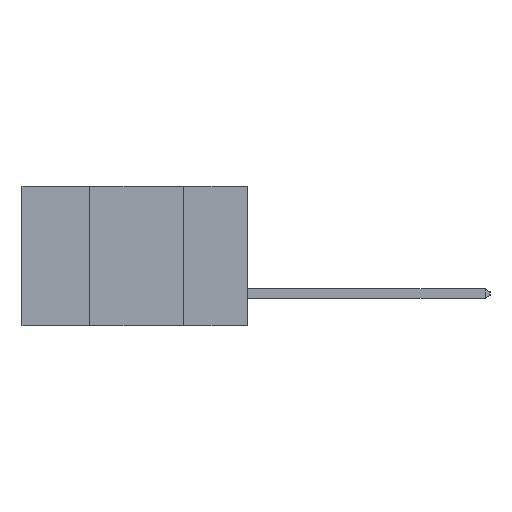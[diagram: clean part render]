
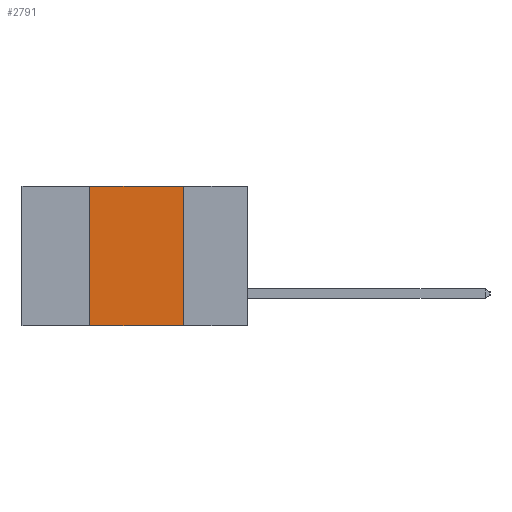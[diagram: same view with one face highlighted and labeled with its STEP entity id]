
A CAD part, left-side view. The second image highlights one B-rep face of the part: STEP entity #2791.
In plain terms, the highlighted planar face has unit normal (-1, 0, 0).
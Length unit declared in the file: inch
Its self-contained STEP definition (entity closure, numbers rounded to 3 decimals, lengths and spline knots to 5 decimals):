
#1742 = CARTESIAN_POINT ( 'NONE',  ( 0., 0.6, 0. ) ) ;
#1952 = ORIENTED_EDGE ( 'NONE', *, *, #18588, .F. ) ;
#2791 = ADVANCED_FACE ( 'NONE', ( #20712 ), #13685, .F. ) ;
#3406 = LINE ( 'NONE', #10914, #11964 ) ;
#4658 = EDGE_CURVE ( 'NONE', #15709, #16392, #15231, .T. ) ;
#6095 = EDGE_CURVE ( 'NONE', #9478, #14396, #9976, .T. ) ;
#6897 = CARTESIAN_POINT ( 'NONE',  ( 0., 0.42, -0.37 ) ) ;
#7161 = DIRECTION ( 'NONE',  ( 0., 0., -1. ) ) ;
#7363 = ORIENTED_EDGE ( 'NONE', *, *, #6095, .F. ) ;
#7579 = CARTESIAN_POINT ( 'NONE',  ( 0., 0.17, -0.37 ) ) ;
#8181 = ORIENTED_EDGE ( 'NONE', *, *, #4658, .F. ) ;
#9433 = EDGE_LOOP ( 'NONE', ( #8181, #1952, #7363, #18022 ) ) ;
#9478 = VERTEX_POINT ( 'NONE', #6897 ) ;
#9529 = VECTOR ( 'NONE', #13599, 39.37008 ) ;
#9976 = LINE ( 'NONE', #10579, #10504 ) ;
#10052 = LINE ( 'NONE', #1742, #9529 ) ;
#10504 = VECTOR ( 'NONE', #10515, 39.37008 ) ;
#10515 = DIRECTION ( 'NONE',  ( 0., 0., 1. ) ) ;
#10579 = CARTESIAN_POINT ( 'NONE',  ( 0., 0.42, -0.37 ) ) ;
#10841 = VECTOR ( 'NONE', #7161, 39.37008 ) ;
#10914 = CARTESIAN_POINT ( 'NONE',  ( 0., 0.6, -0.37 ) ) ;
#11964 = VECTOR ( 'NONE', #12591, 39.37008 ) ;
#12344 = CARTESIAN_POINT ( 'NONE',  ( 0., 0.17, -0.37 ) ) ;
#12591 = DIRECTION ( 'NONE',  ( 0., -1., 0. ) ) ;
#13599 = DIRECTION ( 'NONE',  ( 0., -1., 0. ) ) ;
#13621 = DIRECTION ( 'NONE',  ( 0., 0., -1. ) ) ;
#13624 = DIRECTION ( 'NONE',  ( 1., 0., 0. ) ) ;
#13643 = EDGE_CURVE ( 'NONE', #9478, #16392, #3406, .T. ) ;
#13685 = PLANE ( 'NONE',  #20769 ) ;
#13850 = CARTESIAN_POINT ( 'NONE',  ( 0., 0.6, 0. ) ) ;
#14396 = VERTEX_POINT ( 'NONE', #16378 ) ;
#15231 = LINE ( 'NONE', #7579, #10841 ) ;
#15709 = VERTEX_POINT ( 'NONE', #20413 ) ;
#16378 = CARTESIAN_POINT ( 'NONE',  ( 0., 0.42, 0. ) ) ;
#16392 = VERTEX_POINT ( 'NONE', #12344 ) ;
#18022 = ORIENTED_EDGE ( 'NONE', *, *, #13643, .T. ) ;
#18588 = EDGE_CURVE ( 'NONE', #14396, #15709, #10052, .T. ) ;
#20413 = CARTESIAN_POINT ( 'NONE',  ( 0., 0.17, 0. ) ) ;
#20712 = FACE_OUTER_BOUND ( 'NONE', #9433, .T. ) ;
#20769 = AXIS2_PLACEMENT_3D ( 'NONE', #13850, #13624, #13621 ) ;
